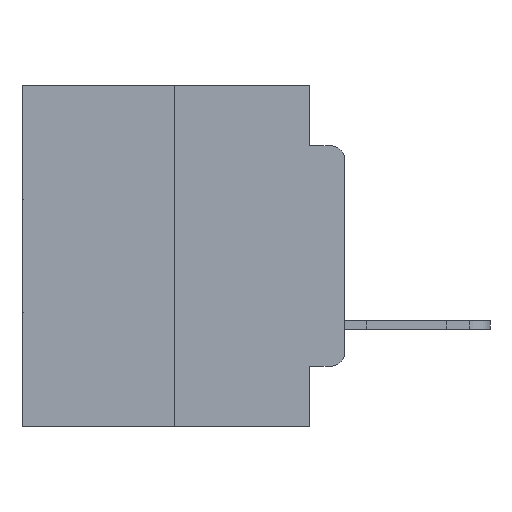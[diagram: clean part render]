
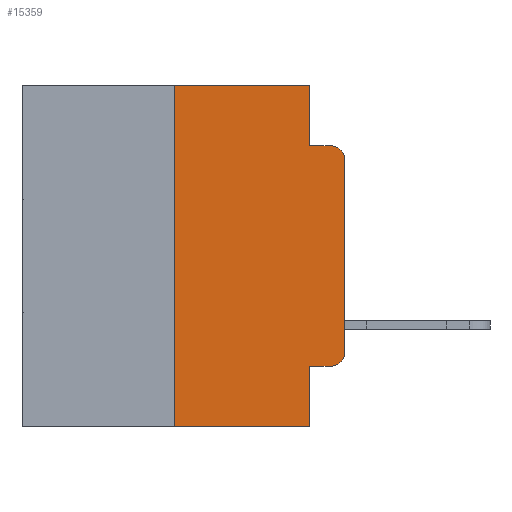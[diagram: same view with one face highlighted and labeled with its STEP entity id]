
A CAD part, left-side view. The second image highlights one B-rep face of the part: STEP entity #15359.
In plain terms, the highlighted planar face has unit normal (-1, 0, 0).
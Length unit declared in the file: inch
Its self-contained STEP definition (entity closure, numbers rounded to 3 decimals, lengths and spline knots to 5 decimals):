
#725 = ORIENTED_EDGE ( 'NONE', *, *, #17286, .F. ) ;
#830 = DIRECTION ( 'NONE',  ( 0., 0., -1. ) ) ;
#878 = DIRECTION ( 'NONE',  ( 1., 0., 0. ) ) ;
#941 = CARTESIAN_POINT ( 'NONE',  ( 0., 0.473, 0. ) ) ;
#1037 = ORIENTED_EDGE ( 'NONE', *, *, #16011, .T. ) ;
#1066 = ORIENTED_EDGE ( 'NONE', *, *, #10098, .F. ) ;
#1168 = PLANE ( 'NONE',  #19769 ) ;
#1659 = VERTEX_POINT ( 'NONE', #23123 ) ;
#2219 = ORIENTED_EDGE ( 'NONE', *, *, #14557, .T. ) ;
#2245 = EDGE_CURVE ( 'NONE', #18754, #18266, #25738, .T. ) ;
#3150 = ORIENTED_EDGE ( 'NONE', *, *, #8608, .T. ) ;
#3232 = EDGE_CURVE ( 'NONE', #17063, #5249, #7140, .T. ) ;
#3291 = CARTESIAN_POINT ( 'NONE',  ( 0., 0.051, 0. ) ) ;
#3827 = CARTESIAN_POINT ( 'NONE',  ( 0., 0., -0.3915 ) ) ;
#4473 = EDGE_LOOP ( 'NONE', ( #13336, #3150, #1066, #6658, #6571, #725, #1037, #5904, #2219, #6694 ) ) ;
#5249 = VERTEX_POINT ( 'NONE', #3291 ) ;
#5506 = CARTESIAN_POINT ( 'NONE',  ( 0., 0.473, 0. ) ) ;
#5904 = ORIENTED_EDGE ( 'NONE', *, *, #15967, .F. ) ;
#5966 = CARTESIAN_POINT ( 'NONE',  ( 0., 0.02, -0.0885 ) ) ;
#6571 = ORIENTED_EDGE ( 'NONE', *, *, #3232, .F. ) ;
#6658 = ORIENTED_EDGE ( 'NONE', *, *, #11630, .F. ) ;
#6694 = ORIENTED_EDGE ( 'NONE', *, *, #13067, .T. ) ;
#7140 = LINE ( 'NONE', #5506, #27596 ) ;
#7309 = AXIS2_PLACEMENT_3D ( 'NONE', #23688, #23628, #23592 ) ;
#7312 = LINE ( 'NONE', #17859, #12569 ) ;
#7464 = CIRCLE ( 'NONE', #7309, 0.02 ) ;
#8608 = EDGE_CURVE ( 'NONE', #18266, #24368, #20855, .T. ) ;
#8866 = CARTESIAN_POINT ( 'NONE',  ( 0., 0.25, 0. ) ) ;
#9530 = LINE ( 'NONE', #18904, #10257 ) ;
#9701 = DIRECTION ( 'NONE',  ( 0., 0., 1. ) ) ;
#10098 = EDGE_CURVE ( 'NONE', #14751, #24368, #16613, .T. ) ;
#10220 = DIRECTION ( 'NONE',  ( 0., -1., 0. ) ) ;
#10257 = VECTOR ( 'NONE', #19150, 39.37008 ) ;
#11475 = VECTOR ( 'NONE', #15016, 39.37008 ) ;
#11630 = EDGE_CURVE ( 'NONE', #5249, #14751, #16471, .T. ) ;
#12569 = VECTOR ( 'NONE', #17071, 39.37008 ) ;
#13067 = EDGE_CURVE ( 'NONE', #18349, #18754, #7464, .T. ) ;
#13291 = FACE_OUTER_BOUND ( 'NONE', #4473, .T. ) ;
#13336 = ORIENTED_EDGE ( 'NONE', *, *, #2245, .T. ) ;
#14557 = EDGE_CURVE ( 'NONE', #22207, #18349, #9530, .T. ) ;
#14751 = VERTEX_POINT ( 'NONE', #15029 ) ;
#14918 = CARTESIAN_POINT ( 'NONE',  ( 0., 0.25, 0. ) ) ;
#15016 = DIRECTION ( 'NONE',  ( 0., 0., -1. ) ) ;
#15029 = CARTESIAN_POINT ( 'NONE',  ( 0., 0.051, -0.0885 ) ) ;
#15052 = CARTESIAN_POINT ( 'NONE',  ( 0., 0.051, 0. ) ) ;
#15359 = ADVANCED_FACE ( 'NONE', ( #13291 ), #1168, .F. ) ;
#15967 = EDGE_CURVE ( 'NONE', #22207, #18089, #19426, .T. ) ;
#16011 = EDGE_CURVE ( 'NONE', #1659, #18089, #7312, .T. ) ;
#16471 = LINE ( 'NONE', #15052, #11475 ) ;
#16613 = LINE ( 'NONE', #25877, #26439 ) ;
#17063 = VERTEX_POINT ( 'NONE', #14918 ) ;
#17071 = DIRECTION ( 'NONE',  ( 0., -1., 0. ) ) ;
#17286 = EDGE_CURVE ( 'NONE', #1659, #17063, #23798, .T. ) ;
#17859 = CARTESIAN_POINT ( 'NONE',  ( 0., 0.473, -0.5 ) ) ;
#18074 = CARTESIAN_POINT ( 'NONE',  ( 0., 0.051, 0. ) ) ;
#18089 = VERTEX_POINT ( 'NONE', #25493 ) ;
#18162 = DIRECTION ( 'NONE',  ( 0., 0., -1. ) ) ;
#18240 = AXIS2_PLACEMENT_3D ( 'NONE', #21730, #21873, #22116 ) ;
#18266 = VERTEX_POINT ( 'NONE', #22196 ) ;
#18349 = VERTEX_POINT ( 'NONE', #20311 ) ;
#18489 = VECTOR ( 'NONE', #9701, 39.37008 ) ;
#18754 = VERTEX_POINT ( 'NONE', #3827 ) ;
#18904 = CARTESIAN_POINT ( 'NONE',  ( 0., 0.051, -0.4115 ) ) ;
#19150 = DIRECTION ( 'NONE',  ( 0., -1., 0. ) ) ;
#19426 = LINE ( 'NONE', #18074, #24706 ) ;
#19769 = AXIS2_PLACEMENT_3D ( 'NONE', #941, #878, #830 ) ;
#19894 = CARTESIAN_POINT ( 'NONE',  ( 0., 0., 0. ) ) ;
#20311 = CARTESIAN_POINT ( 'NONE',  ( 0., 0.02, -0.4115 ) ) ;
#20431 = DIRECTION ( 'NONE',  ( 0., 0., 1. ) ) ;
#20566 = VECTOR ( 'NONE', #20431, 39.37008 ) ;
#20855 = CIRCLE ( 'NONE', #18240, 0.02 ) ;
#21730 = CARTESIAN_POINT ( 'NONE',  ( 0., 0.02, -0.1085 ) ) ;
#21873 = DIRECTION ( 'NONE',  ( -1., 0., 0. ) ) ;
#22116 = DIRECTION ( 'NONE',  ( 0., 0., -1. ) ) ;
#22196 = CARTESIAN_POINT ( 'NONE',  ( 0., 0., -0.1085 ) ) ;
#22207 = VERTEX_POINT ( 'NONE', #25229 ) ;
#23123 = CARTESIAN_POINT ( 'NONE',  ( 0., 0.25, -0.5 ) ) ;
#23592 = DIRECTION ( 'NONE',  ( 0., 0., -1. ) ) ;
#23628 = DIRECTION ( 'NONE',  ( -1., 0., 0. ) ) ;
#23688 = CARTESIAN_POINT ( 'NONE',  ( 0., 0.02, -0.3915 ) ) ;
#23798 = LINE ( 'NONE', #8866, #18489 ) ;
#24368 = VERTEX_POINT ( 'NONE', #5966 ) ;
#24706 = VECTOR ( 'NONE', #18162, 39.37008 ) ;
#25229 = CARTESIAN_POINT ( 'NONE',  ( 0., 0.051, -0.4115 ) ) ;
#25493 = CARTESIAN_POINT ( 'NONE',  ( 0., 0.051, -0.5 ) ) ;
#25625 = DIRECTION ( 'NONE',  ( 0., -1., 0. ) ) ;
#25738 = LINE ( 'NONE', #19894, #20566 ) ;
#25877 = CARTESIAN_POINT ( 'NONE',  ( 0., 0.051, -0.0885 ) ) ;
#26439 = VECTOR ( 'NONE', #25625, 39.37008 ) ;
#27596 = VECTOR ( 'NONE', #10220, 39.37008 ) ;
